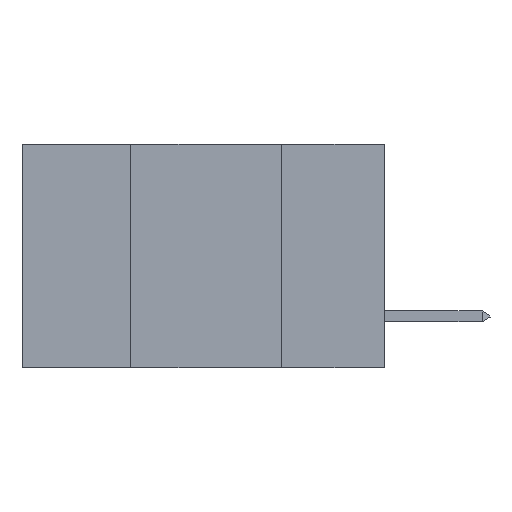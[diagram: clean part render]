
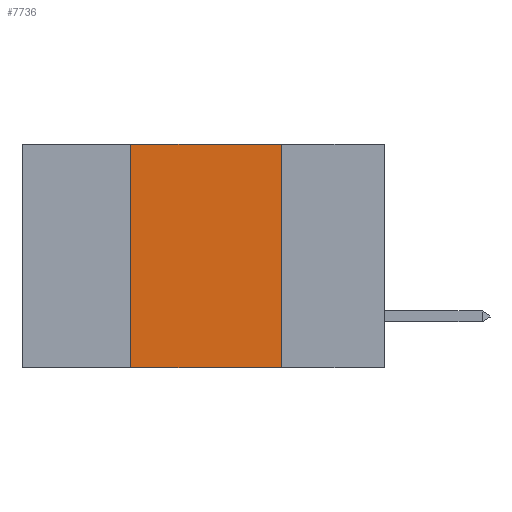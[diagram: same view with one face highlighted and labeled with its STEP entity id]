
A CAD part, left-side view. The second image highlights one B-rep face of the part: STEP entity #7736.
In plain terms, the highlighted planar face has unit normal (-1, 0, 0).
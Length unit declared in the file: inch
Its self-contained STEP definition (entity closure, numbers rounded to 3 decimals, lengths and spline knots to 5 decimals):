
#143 = DIRECTION ( 'NONE',  ( 0., 0., -1. ) ) ;
#1143 = VECTOR ( 'NONE', #2841, 39.37008 ) ;
#2141 = CARTESIAN_POINT ( 'NONE',  ( 0., 0.17, 0. ) ) ;
#2211 = ORIENTED_EDGE ( 'NONE', *, *, #11917, .T. ) ;
#2834 = CARTESIAN_POINT ( 'NONE',  ( 0., 0.17, 0. ) ) ;
#2841 = DIRECTION ( 'NONE',  ( 0., -1., 0. ) ) ;
#2920 = DIRECTION ( 'NONE',  ( 0., -1., 0. ) ) ;
#3076 = AXIS2_PLACEMENT_3D ( 'NONE', #12880, #9084, #143 ) ;
#3451 = VECTOR ( 'NONE', #12472, 39.37008 ) ;
#4870 = LINE ( 'NONE', #2141, #3451 ) ;
#5392 = CARTESIAN_POINT ( 'NONE',  ( 0., 0.6, 0. ) ) ;
#5776 = LINE ( 'NONE', #5392, #12119 ) ;
#6403 = ORIENTED_EDGE ( 'NONE', *, *, #15994, .F. ) ;
#7185 = CARTESIAN_POINT ( 'NONE',  ( 0., 0.42, -0.37 ) ) ;
#7736 = ADVANCED_FACE ( 'NONE', ( #9656 ), #15367, .F. ) ;
#7853 = VERTEX_POINT ( 'NONE', #15669 ) ;
#9084 = DIRECTION ( 'NONE',  ( 1., 0., 0. ) ) ;
#9656 = FACE_OUTER_BOUND ( 'NONE', #10059, .T. ) ;
#9673 = VERTEX_POINT ( 'NONE', #2834 ) ;
#10059 = EDGE_LOOP ( 'NONE', ( #6403, #12212, #14563, #2211 ) ) ;
#11211 = VERTEX_POINT ( 'NONE', #7185 ) ;
#11667 = CARTESIAN_POINT ( 'NONE',  ( 0., 0.6, -0.37 ) ) ;
#11849 = EDGE_CURVE ( 'NONE', #13276, #9673, #5776, .T. ) ;
#11917 = EDGE_CURVE ( 'NONE', #11211, #7853, #14630, .T. ) ;
#12119 = VECTOR ( 'NONE', #2920, 39.37008 ) ;
#12212 = ORIENTED_EDGE ( 'NONE', *, *, #11849, .F. ) ;
#12408 = CARTESIAN_POINT ( 'NONE',  ( 0., 0.42, 0. ) ) ;
#12459 = DIRECTION ( 'NONE',  ( 0., 0., 1. ) ) ;
#12472 = DIRECTION ( 'NONE',  ( 0., 0., -1. ) ) ;
#12880 = CARTESIAN_POINT ( 'NONE',  ( 0., 0.6, 0. ) ) ;
#13276 = VERTEX_POINT ( 'NONE', #13882 ) ;
#13374 = VECTOR ( 'NONE', #12459, 39.37008 ) ;
#13882 = CARTESIAN_POINT ( 'NONE',  ( 0., 0.42, 0. ) ) ;
#13947 = LINE ( 'NONE', #12408, #13374 ) ;
#14563 = ORIENTED_EDGE ( 'NONE', *, *, #15849, .F. ) ;
#14630 = LINE ( 'NONE', #11667, #1143 ) ;
#15367 = PLANE ( 'NONE',  #3076 ) ;
#15669 = CARTESIAN_POINT ( 'NONE',  ( 0., 0.17, -0.37 ) ) ;
#15849 = EDGE_CURVE ( 'NONE', #11211, #13276, #13947, .T. ) ;
#15994 = EDGE_CURVE ( 'NONE', #9673, #7853, #4870, .T. ) ;
